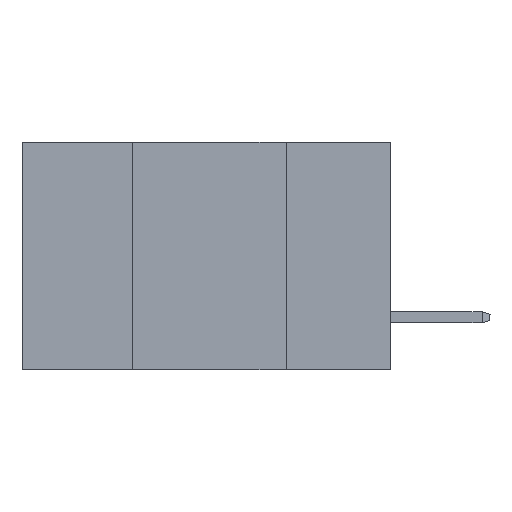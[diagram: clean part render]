
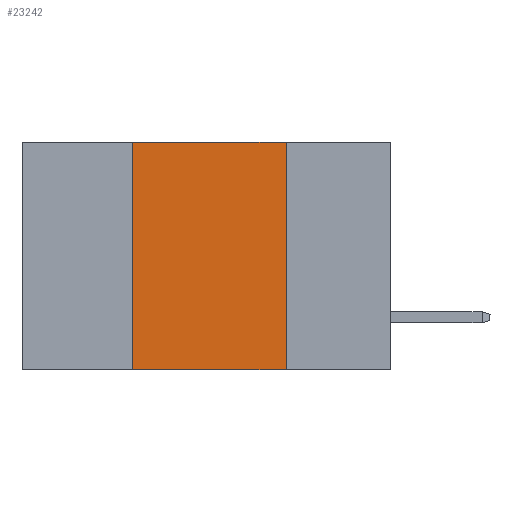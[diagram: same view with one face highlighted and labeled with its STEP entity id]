
A CAD part, left-side view. The second image highlights one B-rep face of the part: STEP entity #23242.
In plain terms, the highlighted planar face has unit normal (-1, 0, 0).
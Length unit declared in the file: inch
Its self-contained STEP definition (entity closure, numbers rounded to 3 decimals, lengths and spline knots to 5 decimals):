
#194 = DIRECTION ( 'NONE',  ( 0., -1., 0. ) ) ;
#661 = VERTEX_POINT ( 'NONE', #13407 ) ;
#911 = LINE ( 'NONE', #22103, #12103 ) ;
#3215 = PLANE ( 'NONE',  #20122 ) ;
#3670 = ORIENTED_EDGE ( 'NONE', *, *, #4300, .T. ) ;
#3771 = CARTESIAN_POINT ( 'NONE',  ( 0., 0.42, -0.37 ) ) ;
#4300 = EDGE_CURVE ( 'NONE', #23090, #9919, #5475, .T. ) ;
#5475 = LINE ( 'NONE', #9977, #22426 ) ;
#6013 = ORIENTED_EDGE ( 'NONE', *, *, #22364, .F. ) ;
#6653 = VERTEX_POINT ( 'NONE', #11554 ) ;
#6850 = ORIENTED_EDGE ( 'NONE', *, *, #15334, .F. ) ;
#7691 = EDGE_LOOP ( 'NONE', ( #6850, #6013, #22222, #3670 ) ) ;
#8442 = CARTESIAN_POINT ( 'NONE',  ( 0., 0.17, -0.37 ) ) ;
#9068 = CARTESIAN_POINT ( 'NONE',  ( 0., 0.17, 0. ) ) ;
#9333 = CARTESIAN_POINT ( 'NONE',  ( 0., 0.42, 0. ) ) ;
#9919 = VERTEX_POINT ( 'NONE', #8442 ) ;
#9977 = CARTESIAN_POINT ( 'NONE',  ( 0., 0.6, -0.37 ) ) ;
#10306 = VECTOR ( 'NONE', #20408, 39.37008 ) ;
#11287 = EDGE_CURVE ( 'NONE', #23090, #661, #11444, .T. ) ;
#11444 = LINE ( 'NONE', #9333, #10306 ) ;
#11554 = CARTESIAN_POINT ( 'NONE',  ( 0., 0.17, 0. ) ) ;
#11927 = DIRECTION ( 'NONE',  ( 0., -1., 0. ) ) ;
#12103 = VECTOR ( 'NONE', #194, 39.37008 ) ;
#13407 = CARTESIAN_POINT ( 'NONE',  ( 0., 0.42, 0. ) ) ;
#15334 = EDGE_CURVE ( 'NONE', #6653, #9919, #22430, .T. ) ;
#15563 = VECTOR ( 'NONE', #21920, 39.37008 ) ;
#15941 = DIRECTION ( 'NONE',  ( 1., 0., 0. ) ) ;
#17779 = CARTESIAN_POINT ( 'NONE',  ( 0., 0.6, 0. ) ) ;
#20122 = AXIS2_PLACEMENT_3D ( 'NONE', #17779, #15941, #20178 ) ;
#20178 = DIRECTION ( 'NONE',  ( 0., 0., -1. ) ) ;
#20408 = DIRECTION ( 'NONE',  ( 0., 0., 1. ) ) ;
#21753 = FACE_OUTER_BOUND ( 'NONE', #7691, .T. ) ;
#21920 = DIRECTION ( 'NONE',  ( 0., 0., -1. ) ) ;
#22103 = CARTESIAN_POINT ( 'NONE',  ( 0., 0.6, 0. ) ) ;
#22222 = ORIENTED_EDGE ( 'NONE', *, *, #11287, .F. ) ;
#22364 = EDGE_CURVE ( 'NONE', #661, #6653, #911, .T. ) ;
#22426 = VECTOR ( 'NONE', #11927, 39.37008 ) ;
#22430 = LINE ( 'NONE', #9068, #15563 ) ;
#23090 = VERTEX_POINT ( 'NONE', #3771 ) ;
#23242 = ADVANCED_FACE ( 'NONE', ( #21753 ), #3215, .F. ) ;
